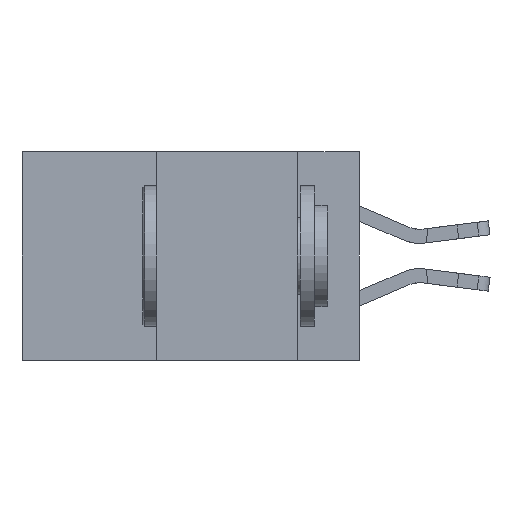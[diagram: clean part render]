
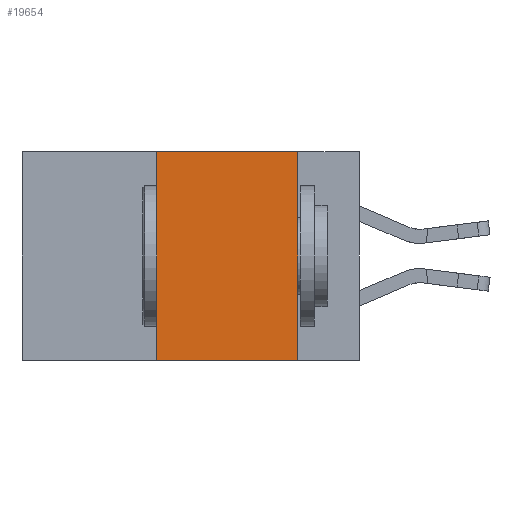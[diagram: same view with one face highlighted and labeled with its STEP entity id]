
A CAD part, left-side view. The second image highlights one B-rep face of the part: STEP entity #19654.
In plain terms, the highlighted planar face has unit normal (-1, 0, 0).
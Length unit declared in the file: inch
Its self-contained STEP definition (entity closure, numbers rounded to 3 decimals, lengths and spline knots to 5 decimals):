
#898 = CARTESIAN_POINT ( 'NONE',  ( 0., 0.11, 0. ) ) ;
#926 = VECTOR ( 'NONE', #3265, 39.37008 ) ;
#1450 = DIRECTION ( 'NONE',  ( 0., 0., -1. ) ) ;
#2259 = LINE ( 'NONE', #9725, #24825 ) ;
#3197 = DIRECTION ( 'NONE',  ( 0., -1., 0. ) ) ;
#3265 = DIRECTION ( 'NONE',  ( 0., 0., -1. ) ) ;
#4982 = VERTEX_POINT ( 'NONE', #23638 ) ;
#5493 = EDGE_CURVE ( 'NONE', #4982, #18792, #26462, .T. ) ;
#6694 = LINE ( 'NONE', #19449, #926 ) ;
#7483 = CARTESIAN_POINT ( 'NONE',  ( 0., 0.6, -0.37 ) ) ;
#7781 = DIRECTION ( 'NONE',  ( 0., -1., 0. ) ) ;
#8235 = EDGE_CURVE ( 'NONE', #27799, #16232, #26448, .T. ) ;
#9725 = CARTESIAN_POINT ( 'NONE',  ( 0., 0.36, 0. ) ) ;
#9820 = CARTESIAN_POINT ( 'NONE',  ( 0., 0.11, -0.37 ) ) ;
#11178 = FACE_OUTER_BOUND ( 'NONE', #26352, .T. ) ;
#12313 = CARTESIAN_POINT ( 'NONE',  ( 0., 0.36, -0.37 ) ) ;
#12639 = EDGE_CURVE ( 'NONE', #27799, #4982, #2259, .T. ) ;
#13028 = AXIS2_PLACEMENT_3D ( 'NONE', #27589, #14507, #1450 ) ;
#14142 = VECTOR ( 'NONE', #7781, 39.37008 ) ;
#14507 = DIRECTION ( 'NONE',  ( 1., 0., 0. ) ) ;
#16232 = VERTEX_POINT ( 'NONE', #9820 ) ;
#18513 = EDGE_CURVE ( 'NONE', #18792, #16232, #6694, .T. ) ;
#18616 = CARTESIAN_POINT ( 'NONE',  ( 0., 0.6, 0. ) ) ;
#18792 = VERTEX_POINT ( 'NONE', #898 ) ;
#19449 = CARTESIAN_POINT ( 'NONE',  ( 0., 0.11, 0. ) ) ;
#19654 = ADVANCED_FACE ( 'NONE', ( #11178 ), #21026, .F. ) ;
#20643 = VECTOR ( 'NONE', #3197, 39.37008 ) ;
#21026 = PLANE ( 'NONE',  #13028 ) ;
#22410 = ORIENTED_EDGE ( 'NONE', *, *, #18513, .F. ) ;
#23204 = ORIENTED_EDGE ( 'NONE', *, *, #5493, .F. ) ;
#23638 = CARTESIAN_POINT ( 'NONE',  ( 0., 0.36, 0. ) ) ;
#24420 = ORIENTED_EDGE ( 'NONE', *, *, #12639, .F. ) ;
#24825 = VECTOR ( 'NONE', #27207, 39.37008 ) ;
#25163 = ORIENTED_EDGE ( 'NONE', *, *, #8235, .T. ) ;
#26352 = EDGE_LOOP ( 'NONE', ( #22410, #23204, #24420, #25163 ) ) ;
#26448 = LINE ( 'NONE', #7483, #20643 ) ;
#26462 = LINE ( 'NONE', #18616, #14142 ) ;
#27207 = DIRECTION ( 'NONE',  ( 0., 0., 1. ) ) ;
#27589 = CARTESIAN_POINT ( 'NONE',  ( 0., 0.6, 0. ) ) ;
#27799 = VERTEX_POINT ( 'NONE', #12313 ) ;
